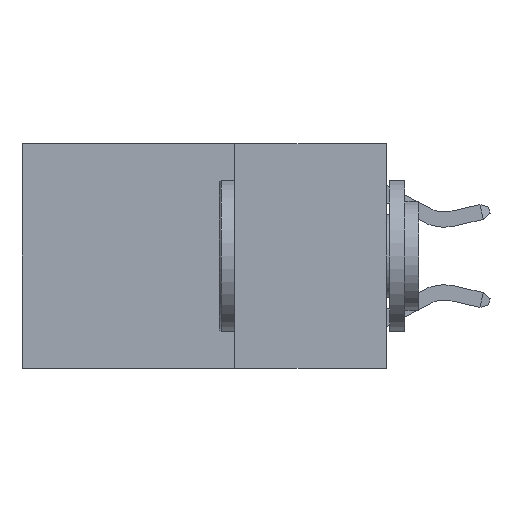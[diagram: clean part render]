
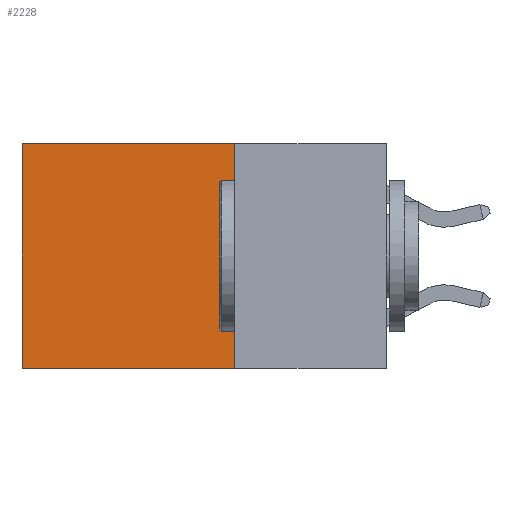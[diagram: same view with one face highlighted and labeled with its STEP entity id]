
A CAD part, left-side view. The second image highlights one B-rep face of the part: STEP entity #2228.
In plain terms, the highlighted planar face has unit normal (-1, 0, 0).
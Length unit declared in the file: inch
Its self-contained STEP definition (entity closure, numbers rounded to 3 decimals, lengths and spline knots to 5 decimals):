
#154 = VECTOR ( 'NONE', #15896, 39.37008 ) ;
#1022 = CARTESIAN_POINT ( 'NONE',  ( 0.2625, 0.25, 0. ) ) ;
#1448 = VERTEX_POINT ( 'NONE', #3997 ) ;
#1866 = VECTOR ( 'NONE', #4165, 39.37008 ) ;
#2228 = ADVANCED_FACE ( 'NONE', ( #12312 ), #8739, .F. ) ;
#2997 = CARTESIAN_POINT ( 'NONE',  ( 0.2625, 0.25, 0. ) ) ;
#3229 = EDGE_LOOP ( 'NONE', ( #5479, #10178, #14955, #13884 ) ) ;
#3869 = CARTESIAN_POINT ( 'NONE',  ( 0.2625, 0.25, 0. ) ) ;
#3890 = EDGE_CURVE ( 'NONE', #10437, #16163, #11334, .T. ) ;
#3997 = CARTESIAN_POINT ( 'NONE',  ( 0.2625, 0.6, 0. ) ) ;
#4165 = DIRECTION ( 'NONE',  ( 0., 0., -1. ) ) ;
#4346 = VECTOR ( 'NONE', #14059, 39.37008 ) ;
#5479 = ORIENTED_EDGE ( 'NONE', *, *, #7869, .T. ) ;
#6158 = DIRECTION ( 'NONE',  ( 1., 0., 0. ) ) ;
#6861 = EDGE_CURVE ( 'NONE', #9182, #10437, #14087, .T. ) ;
#7106 = CARTESIAN_POINT ( 'NONE',  ( 0.2625, 0.6, -0.37 ) ) ;
#7341 = DIRECTION ( 'NONE',  ( 0., 0., -1. ) ) ;
#7869 = EDGE_CURVE ( 'NONE', #1448, #16163, #13197, .T. ) ;
#8739 = PLANE ( 'NONE',  #13286 ) ;
#9182 = VERTEX_POINT ( 'NONE', #15833 ) ;
#9806 = DIRECTION ( 'NONE',  ( 0., 1., 0. ) ) ;
#10178 = ORIENTED_EDGE ( 'NONE', *, *, #3890, .F. ) ;
#10437 = VERTEX_POINT ( 'NONE', #12226 ) ;
#11334 = LINE ( 'NONE', #16250, #12548 ) ;
#11774 = EDGE_CURVE ( 'NONE', #9182, #1448, #15431, .T. ) ;
#12226 = CARTESIAN_POINT ( 'NONE',  ( 0.2625, 0.25, -0.37 ) ) ;
#12312 = FACE_OUTER_BOUND ( 'NONE', #3229, .T. ) ;
#12548 = VECTOR ( 'NONE', #9806, 39.37008 ) ;
#13197 = LINE ( 'NONE', #14602, #154 ) ;
#13286 = AXIS2_PLACEMENT_3D ( 'NONE', #1022, #6158, #7341 ) ;
#13884 = ORIENTED_EDGE ( 'NONE', *, *, #11774, .T. ) ;
#14059 = DIRECTION ( 'NONE',  ( 0., 1., 0. ) ) ;
#14087 = LINE ( 'NONE', #2997, #1866 ) ;
#14602 = CARTESIAN_POINT ( 'NONE',  ( 0.2625, 0.6, 0. ) ) ;
#14955 = ORIENTED_EDGE ( 'NONE', *, *, #6861, .F. ) ;
#15431 = LINE ( 'NONE', #3869, #4346 ) ;
#15833 = CARTESIAN_POINT ( 'NONE',  ( 0.2625, 0.25, 0. ) ) ;
#15896 = DIRECTION ( 'NONE',  ( 0., 0., -1. ) ) ;
#16163 = VERTEX_POINT ( 'NONE', #7106 ) ;
#16250 = CARTESIAN_POINT ( 'NONE',  ( 0.2625, 0.25, -0.37 ) ) ;
